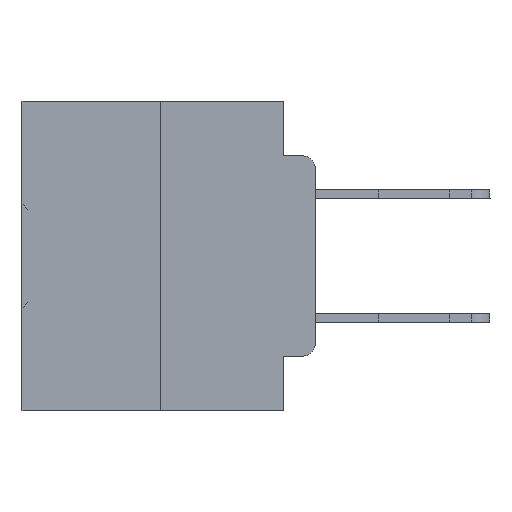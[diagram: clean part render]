
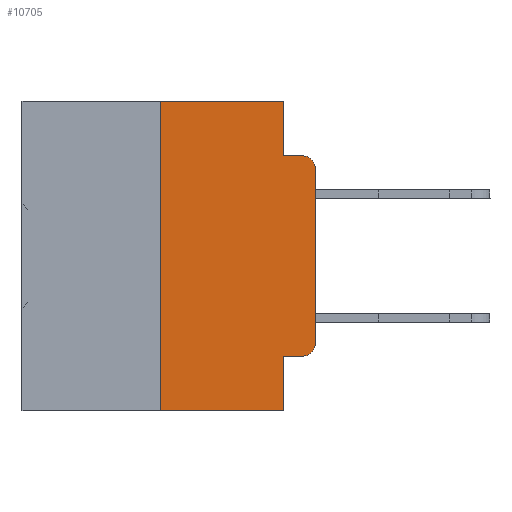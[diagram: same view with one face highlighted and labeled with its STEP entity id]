
A CAD part, left-side view. The second image highlights one B-rep face of the part: STEP entity #10705.
In plain terms, the highlighted planar face has unit normal (-1, 0, 0).
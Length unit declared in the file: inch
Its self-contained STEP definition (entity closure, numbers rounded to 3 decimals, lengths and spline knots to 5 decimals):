
#268 = EDGE_CURVE ( 'NONE', #31658, #12434, #11537, .T. ) ;
#843 = CARTESIAN_POINT ( 'NONE',  ( 0., 0.051, -0.0885 ) ) ;
#1152 = ORIENTED_EDGE ( 'NONE', *, *, #12657, .F. ) ;
#2483 = AXIS2_PLACEMENT_3D ( 'NONE', #7724, #18821, #33719 ) ;
#2916 = VERTEX_POINT ( 'NONE', #6371 ) ;
#3251 = VERTEX_POINT ( 'NONE', #6283 ) ;
#3301 = VECTOR ( 'NONE', #26943, 39.37008 ) ;
#3420 = CARTESIAN_POINT ( 'NONE',  ( 0., 0.02, -0.3915 ) ) ;
#3493 = CARTESIAN_POINT ( 'NONE',  ( 0., 0.051, -0.4115 ) ) ;
#4425 = ORIENTED_EDGE ( 'NONE', *, *, #268, .T. ) ;
#5242 = LINE ( 'NONE', #17485, #12208 ) ;
#5490 = AXIS2_PLACEMENT_3D ( 'NONE', #3420, #35545, #18158 ) ;
#5621 = CARTESIAN_POINT ( 'NONE',  ( 0., 0., -0.1085 ) ) ;
#5636 = CARTESIAN_POINT ( 'NONE',  ( 0., 0.02, -0.4115 ) ) ;
#5895 = EDGE_CURVE ( 'NONE', #3251, #24701, #5242, .T. ) ;
#5998 = VERTEX_POINT ( 'NONE', #5621 ) ;
#6089 = CIRCLE ( 'NONE', #5490, 0.02 ) ;
#6211 = ORIENTED_EDGE ( 'NONE', *, *, #31295, .T. ) ;
#6283 = CARTESIAN_POINT ( 'NONE',  ( 0., 0.25, -0.5 ) ) ;
#6311 = ORIENTED_EDGE ( 'NONE', *, *, #22178, .F. ) ;
#6371 = CARTESIAN_POINT ( 'NONE',  ( 0., 0.051, 0. ) ) ;
#7312 = DIRECTION ( 'NONE',  ( 0., 0., 1. ) ) ;
#7438 = VERTEX_POINT ( 'NONE', #32771 ) ;
#7617 = VERTEX_POINT ( 'NONE', #19942 ) ;
#7724 = CARTESIAN_POINT ( 'NONE',  ( 0., 0.02, -0.1085 ) ) ;
#7793 = CARTESIAN_POINT ( 'NONE',  ( 0., 0.473, 0. ) ) ;
#10705 = ADVANCED_FACE ( 'NONE', ( #34546 ), #22712, .F. ) ;
#10722 = EDGE_CURVE ( 'NONE', #24701, #2916, #22332, .T. ) ;
#11222 = DIRECTION ( 'NONE',  ( 0., -1., 0. ) ) ;
#11537 = LINE ( 'NONE', #3493, #24788 ) ;
#11726 = EDGE_CURVE ( 'NONE', #24211, #11740, #12415, .T. ) ;
#11740 = VERTEX_POINT ( 'NONE', #23501 ) ;
#12208 = VECTOR ( 'NONE', #37167, 39.37008 ) ;
#12415 = LINE ( 'NONE', #26565, #3301 ) ;
#12434 = VERTEX_POINT ( 'NONE', #5636 ) ;
#12657 = EDGE_CURVE ( 'NONE', #2916, #24211, #27411, .T. ) ;
#13539 = DIRECTION ( 'NONE',  ( 1., 0., 0. ) ) ;
#13557 = CARTESIAN_POINT ( 'NONE',  ( 0., 0.051, 0. ) ) ;
#15010 = VECTOR ( 'NONE', #33709, 39.37008 ) ;
#17485 = CARTESIAN_POINT ( 'NONE',  ( 0., 0.25, 0. ) ) ;
#17680 = VECTOR ( 'NONE', #19464, 39.37008 ) ;
#17991 = EDGE_LOOP ( 'NONE', ( #6211, #27911, #18417, #1152, #30120, #26031, #23014, #6311, #4425, #29289 ) ) ;
#18158 = DIRECTION ( 'NONE',  ( 0., 0., -1. ) ) ;
#18417 = ORIENTED_EDGE ( 'NONE', *, *, #11726, .F. ) ;
#18590 = EDGE_CURVE ( 'NONE', #5998, #11740, #35461, .T. ) ;
#18623 = CARTESIAN_POINT ( 'NONE',  ( 0., 0.051, 0. ) ) ;
#18821 = DIRECTION ( 'NONE',  ( -1., 0., 0. ) ) ;
#19464 = DIRECTION ( 'NONE',  ( 0., -1., 0. ) ) ;
#19942 = CARTESIAN_POINT ( 'NONE',  ( 0., 0., -0.3915 ) ) ;
#20212 = CARTESIAN_POINT ( 'NONE',  ( 0., 0.473, 0. ) ) ;
#20330 = VECTOR ( 'NONE', #30580, 39.37008 ) ;
#21781 = LINE ( 'NONE', #13557, #20330 ) ;
#21843 = CARTESIAN_POINT ( 'NONE',  ( 0., 0., 0. ) ) ;
#22178 = EDGE_CURVE ( 'NONE', #31658, #7438, #21781, .T. ) ;
#22332 = LINE ( 'NONE', #20212, #17680 ) ;
#22712 = PLANE ( 'NONE',  #23164 ) ;
#23014 = ORIENTED_EDGE ( 'NONE', *, *, #32267, .T. ) ;
#23164 = AXIS2_PLACEMENT_3D ( 'NONE', #7793, #13539, #28621 ) ;
#23501 = CARTESIAN_POINT ( 'NONE',  ( 0., 0.02, -0.0885 ) ) ;
#24211 = VERTEX_POINT ( 'NONE', #843 ) ;
#24701 = VERTEX_POINT ( 'NONE', #30448 ) ;
#24788 = VECTOR ( 'NONE', #31817, 39.37008 ) ;
#25762 = LINE ( 'NONE', #37407, #37312 ) ;
#26031 = ORIENTED_EDGE ( 'NONE', *, *, #5895, .F. ) ;
#26565 = CARTESIAN_POINT ( 'NONE',  ( 0., 0.051, -0.0885 ) ) ;
#26943 = DIRECTION ( 'NONE',  ( 0., -1., 0. ) ) ;
#27411 = LINE ( 'NONE', #18623, #15010 ) ;
#27911 = ORIENTED_EDGE ( 'NONE', *, *, #18590, .T. ) ;
#27915 = CARTESIAN_POINT ( 'NONE',  ( 0., 0.051, -0.4115 ) ) ;
#28621 = DIRECTION ( 'NONE',  ( 0., 0., -1. ) ) ;
#29289 = ORIENTED_EDGE ( 'NONE', *, *, #29457, .T. ) ;
#29457 = EDGE_CURVE ( 'NONE', #12434, #7617, #6089, .T. ) ;
#30120 = ORIENTED_EDGE ( 'NONE', *, *, #10722, .F. ) ;
#30448 = CARTESIAN_POINT ( 'NONE',  ( 0., 0.25, 0. ) ) ;
#30580 = DIRECTION ( 'NONE',  ( 0., 0., -1. ) ) ;
#31295 = EDGE_CURVE ( 'NONE', #7617, #5998, #36370, .T. ) ;
#31658 = VERTEX_POINT ( 'NONE', #27915 ) ;
#31817 = DIRECTION ( 'NONE',  ( 0., -1., 0. ) ) ;
#32267 = EDGE_CURVE ( 'NONE', #3251, #7438, #25762, .T. ) ;
#32771 = CARTESIAN_POINT ( 'NONE',  ( 0., 0.051, -0.5 ) ) ;
#33709 = DIRECTION ( 'NONE',  ( 0., 0., -1. ) ) ;
#33719 = DIRECTION ( 'NONE',  ( 0., 0., -1. ) ) ;
#34546 = FACE_OUTER_BOUND ( 'NONE', #17991, .T. ) ;
#34796 = VECTOR ( 'NONE', #7312, 39.37008 ) ;
#35461 = CIRCLE ( 'NONE', #2483, 0.02 ) ;
#35545 = DIRECTION ( 'NONE',  ( -1., 0., 0. ) ) ;
#36370 = LINE ( 'NONE', #21843, #34796 ) ;
#37167 = DIRECTION ( 'NONE',  ( 0., 0., 1. ) ) ;
#37312 = VECTOR ( 'NONE', #11222, 39.37008 ) ;
#37407 = CARTESIAN_POINT ( 'NONE',  ( 0., 0.473, -0.5 ) ) ;
